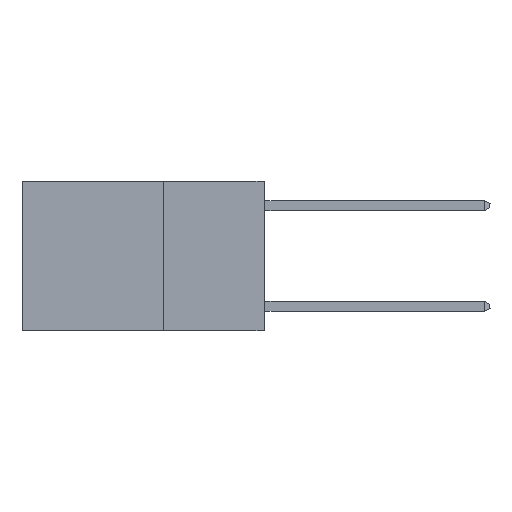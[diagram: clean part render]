
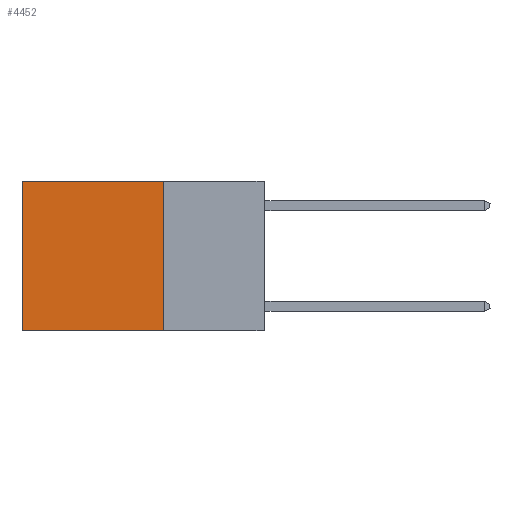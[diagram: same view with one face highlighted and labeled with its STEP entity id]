
A CAD part, left-side view. The second image highlights one B-rep face of the part: STEP entity #4452.
In plain terms, the highlighted planar face has unit normal (-1, 0, 0).
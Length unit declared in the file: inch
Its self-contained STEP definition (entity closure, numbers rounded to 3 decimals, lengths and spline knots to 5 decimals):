
#1511 = DIRECTION ( 'NONE',  ( 1., 0., 0. ) ) ;
#1613 = EDGE_CURVE ( 'NONE', #11934, #10294, #14629, .T. ) ;
#1886 = EDGE_CURVE ( 'NONE', #4058, #9601, #11585, .T. ) ;
#1945 = CARTESIAN_POINT ( 'NONE',  ( 0.2625, 0.6, -0.37 ) ) ;
#2202 = DIRECTION ( 'NONE',  ( 0., 1., 0. ) ) ;
#2784 = LINE ( 'NONE', #12491, #11153 ) ;
#3865 = VECTOR ( 'NONE', #8045, 39.37008 ) ;
#3868 = CARTESIAN_POINT ( 'NONE',  ( 0.2625, 0.6, 0. ) ) ;
#3931 = CARTESIAN_POINT ( 'NONE',  ( 0.2625, 0.25, 0. ) ) ;
#4058 = VERTEX_POINT ( 'NONE', #3868 ) ;
#4352 = CARTESIAN_POINT ( 'NONE',  ( 0.2625, 0.6, 0. ) ) ;
#4452 = ADVANCED_FACE ( 'NONE', ( #12404 ), #12252, .F. ) ;
#5199 = DIRECTION ( 'NONE',  ( 0., 0., -1. ) ) ;
#5595 = ORIENTED_EDGE ( 'NONE', *, *, #1886, .T. ) ;
#5682 = CARTESIAN_POINT ( 'NONE',  ( 0.2625, 0.25, 0. ) ) ;
#7242 = LINE ( 'NONE', #8290, #8219 ) ;
#8045 = DIRECTION ( 'NONE',  ( 0., 0., -1. ) ) ;
#8219 = VECTOR ( 'NONE', #2202, 39.37008 ) ;
#8290 = CARTESIAN_POINT ( 'NONE',  ( 0.2625, 0.25, -0.37 ) ) ;
#8486 = DIRECTION ( 'NONE',  ( 0., 0., -1. ) ) ;
#9514 = VECTOR ( 'NONE', #5199, 39.37008 ) ;
#9601 = VERTEX_POINT ( 'NONE', #1945 ) ;
#10262 = ORIENTED_EDGE ( 'NONE', *, *, #15122, .F. ) ;
#10294 = VERTEX_POINT ( 'NONE', #15655 ) ;
#10353 = EDGE_LOOP ( 'NONE', ( #5595, #10262, #11070, #12844 ) ) ;
#11070 = ORIENTED_EDGE ( 'NONE', *, *, #1613, .F. ) ;
#11153 = VECTOR ( 'NONE', #11371, 39.37008 ) ;
#11371 = DIRECTION ( 'NONE',  ( 0., 1., 0. ) ) ;
#11585 = LINE ( 'NONE', #4352, #3865 ) ;
#11841 = EDGE_CURVE ( 'NONE', #11934, #4058, #2784, .T. ) ;
#11934 = VERTEX_POINT ( 'NONE', #5682 ) ;
#12252 = PLANE ( 'NONE',  #14501 ) ;
#12404 = FACE_OUTER_BOUND ( 'NONE', #10353, .T. ) ;
#12491 = CARTESIAN_POINT ( 'NONE',  ( 0.2625, 0.25, 0. ) ) ;
#12844 = ORIENTED_EDGE ( 'NONE', *, *, #11841, .T. ) ;
#13278 = CARTESIAN_POINT ( 'NONE',  ( 0.2625, 0.25, 0. ) ) ;
#14501 = AXIS2_PLACEMENT_3D ( 'NONE', #13278, #1511, #8486 ) ;
#14629 = LINE ( 'NONE', #3931, #9514 ) ;
#15122 = EDGE_CURVE ( 'NONE', #10294, #9601, #7242, .T. ) ;
#15655 = CARTESIAN_POINT ( 'NONE',  ( 0.2625, 0.25, -0.37 ) ) ;
